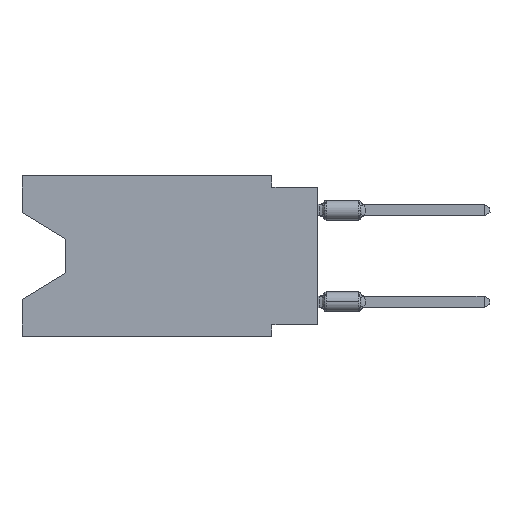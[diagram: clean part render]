
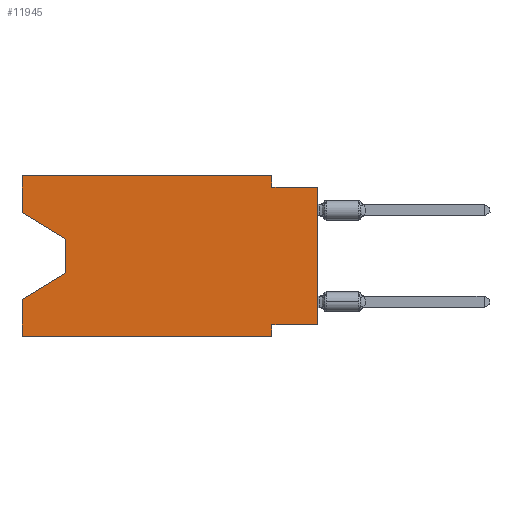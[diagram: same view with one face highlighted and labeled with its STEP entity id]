
A CAD part, left-side view. The second image highlights one B-rep face of the part: STEP entity #11945.
In plain terms, the highlighted planar face has unit normal (-1, 0, 0).
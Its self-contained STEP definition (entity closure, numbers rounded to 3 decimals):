
#227 = VERTEX_POINT ( 'NONE', #22464 ) ;
#343 = VECTOR ( 'NONE', #11981, 1000. ) ;
#1272 = LINE ( 'NONE', #13724, #18395 ) ;
#1464 = CARTESIAN_POINT ( 'NONE',  ( 0., 2.54, -8.255 ) ) ;
#1470 = DIRECTION ( 'NONE',  ( 0., -1., 0. ) ) ;
#1508 = VECTOR ( 'NONE', #5732, 1000. ) ;
#1556 = ORIENTED_EDGE ( 'NONE', *, *, #2219, .F. ) ;
#1916 = EDGE_CURVE ( 'NONE', #15189, #8609, #19212, .T. ) ;
#2058 = LINE ( 'NONE', #9083, #20916 ) ;
#2219 = EDGE_CURVE ( 'NONE', #227, #12542, #18964, .T. ) ;
#2489 = CARTESIAN_POINT ( 'NONE',  ( 0., 2.54, -0.635 ) ) ;
#2504 = LINE ( 'NONE', #8159, #2540 ) ;
#2540 = VECTOR ( 'NONE', #15192, 1000. ) ;
#2694 = VECTOR ( 'NONE', #19600, 1000. ) ;
#3168 = CARTESIAN_POINT ( 'NONE',  ( 0., 16.383, 0. ) ) ;
#3346 = DIRECTION ( 'NONE',  ( 0., 1., 0. ) ) ;
#3397 = DIRECTION ( 'NONE',  ( 0., 0.855, -0.519 ) ) ;
#3561 = CARTESIAN_POINT ( 'NONE',  ( 0., 0., -0.635 ) ) ;
#3777 = CARTESIAN_POINT ( 'NONE',  ( 0., 16.383, -8.89 ) ) ;
#4109 = CARTESIAN_POINT ( 'NONE',  ( 0., 2.54, -8.89 ) ) ;
#4114 = CARTESIAN_POINT ( 'NONE',  ( 0., 16.383, -2.038 ) ) ;
#4242 = CARTESIAN_POINT ( 'NONE',  ( 0., 0., -8.255 ) ) ;
#4996 = VERTEX_POINT ( 'NONE', #4109 ) ;
#5250 = ORIENTED_EDGE ( 'NONE', *, *, #13759, .F. ) ;
#5732 = DIRECTION ( 'NONE',  ( 0., -1., 0. ) ) ;
#5753 = CARTESIAN_POINT ( 'NONE',  ( 0., 16.383, -6.852 ) ) ;
#6162 = CARTESIAN_POINT ( 'NONE',  ( 0., 13.97, -5.385 ) ) ;
#6175 = PLANE ( 'NONE',  #8049 ) ;
#6365 = VERTEX_POINT ( 'NONE', #2489 ) ;
#6407 = DIRECTION ( 'NONE',  ( 0., 0., 1. ) ) ;
#6963 = VECTOR ( 'NONE', #1470, 1000. ) ;
#7028 = LINE ( 'NONE', #21099, #15801 ) ;
#7045 = EDGE_CURVE ( 'NONE', #15189, #11457, #2058, .T. ) ;
#7484 = DIRECTION ( 'NONE',  ( 0., 0., 1. ) ) ;
#7676 = DIRECTION ( 'NONE',  ( 1., 0., 0. ) ) ;
#8006 = CARTESIAN_POINT ( 'NONE',  ( 0., 0., -0.635 ) ) ;
#8049 = AXIS2_PLACEMENT_3D ( 'NONE', #14593, #7676, #16686 ) ;
#8159 = CARTESIAN_POINT ( 'NONE',  ( 0., 2.54, -8.89 ) ) ;
#8609 = VERTEX_POINT ( 'NONE', #9090 ) ;
#9083 = CARTESIAN_POINT ( 'NONE',  ( 0., 16.383, 0. ) ) ;
#9090 = CARTESIAN_POINT ( 'NONE',  ( 0., 13.97, -3.505 ) ) ;
#9149 = CARTESIAN_POINT ( 'NONE',  ( 0., 13.97, -3.505 ) ) ;
#9160 = ORIENTED_EDGE ( 'NONE', *, *, #18349, .T. ) ;
#9406 = LINE ( 'NONE', #3777, #1508 ) ;
#10370 = LINE ( 'NONE', #3561, #343 ) ;
#10727 = LINE ( 'NONE', #21787, #2694 ) ;
#10815 = ORIENTED_EDGE ( 'NONE', *, *, #7045, .F. ) ;
#11188 = EDGE_CURVE ( 'NONE', #11465, #11689, #1272, .T. ) ;
#11203 = EDGE_CURVE ( 'NONE', #6365, #21708, #10370, .T. ) ;
#11457 = VERTEX_POINT ( 'NONE', #20043 ) ;
#11465 = VERTEX_POINT ( 'NONE', #4242 ) ;
#11689 = VERTEX_POINT ( 'NONE', #1464 ) ;
#11945 = ADVANCED_FACE ( 'NONE', ( #13098 ), #6175, .F. ) ;
#11981 = DIRECTION ( 'NONE',  ( 0., -1., 0. ) ) ;
#12382 = EDGE_CURVE ( 'NONE', #17687, #6365, #7028, .T. ) ;
#12542 = VERTEX_POINT ( 'NONE', #5753 ) ;
#12720 = ORIENTED_EDGE ( 'NONE', *, *, #11203, .F. ) ;
#13098 = FACE_OUTER_BOUND ( 'NONE', #14072, .T. ) ;
#13263 = VECTOR ( 'NONE', #3397, 1000. ) ;
#13280 = ORIENTED_EDGE ( 'NONE', *, *, #11188, .F. ) ;
#13308 = VECTOR ( 'NONE', #13913, 1000. ) ;
#13724 = CARTESIAN_POINT ( 'NONE',  ( 0., 0., -8.255 ) ) ;
#13759 = EDGE_CURVE ( 'NONE', #11457, #17687, #15653, .T. ) ;
#13913 = DIRECTION ( 'NONE',  ( 0., -0.855, -0.519 ) ) ;
#14072 = EDGE_LOOP ( 'NONE', ( #15788, #9160, #15141, #1556, #22695, #16688, #13280, #14686, #12720, #17337, #5250, #10815 ) ) ;
#14593 = CARTESIAN_POINT ( 'NONE',  ( 0., 16.383, 0. ) ) ;
#14686 = ORIENTED_EDGE ( 'NONE', *, *, #19198, .T. ) ;
#14922 = DIRECTION ( 'NONE',  ( 0., 0., -1. ) ) ;
#15141 = ORIENTED_EDGE ( 'NONE', *, *, #21899, .T. ) ;
#15189 = VERTEX_POINT ( 'NONE', #4114 ) ;
#15192 = DIRECTION ( 'NONE',  ( 0., 0., -1. ) ) ;
#15242 = EDGE_CURVE ( 'NONE', #227, #4996, #9406, .T. ) ;
#15545 = VECTOR ( 'NONE', #14922, 1000. ) ;
#15653 = LINE ( 'NONE', #20620, #6963 ) ;
#15788 = ORIENTED_EDGE ( 'NONE', *, *, #1916, .T. ) ;
#15801 = VECTOR ( 'NONE', #19021, 1000. ) ;
#15867 = CARTESIAN_POINT ( 'NONE',  ( 0., 16.383, -2.038 ) ) ;
#16327 = LINE ( 'NONE', #9149, #15545 ) ;
#16686 = DIRECTION ( 'NONE',  ( 0., 0., -1. ) ) ;
#16688 = ORIENTED_EDGE ( 'NONE', *, *, #20996, .F. ) ;
#17128 = VERTEX_POINT ( 'NONE', #6162 ) ;
#17282 = CARTESIAN_POINT ( 'NONE',  ( 0., 2.54, 0. ) ) ;
#17337 = ORIENTED_EDGE ( 'NONE', *, *, #12382, .F. ) ;
#17687 = VERTEX_POINT ( 'NONE', #17282 ) ;
#18349 = EDGE_CURVE ( 'NONE', #8609, #17128, #16327, .T. ) ;
#18395 = VECTOR ( 'NONE', #3346, 1000. ) ;
#18520 = VECTOR ( 'NONE', #6407, 1000. ) ;
#18964 = LINE ( 'NONE', #3168, #18520 ) ;
#19021 = DIRECTION ( 'NONE',  ( 0., 0., -1. ) ) ;
#19198 = EDGE_CURVE ( 'NONE', #11465, #21708, #10727, .T. ) ;
#19212 = LINE ( 'NONE', #15867, #13308 ) ;
#19600 = DIRECTION ( 'NONE',  ( 0., 0., 1. ) ) ;
#20043 = CARTESIAN_POINT ( 'NONE',  ( 0., 16.383, 0. ) ) ;
#20579 = CARTESIAN_POINT ( 'NONE',  ( 0., 13.97, -5.385 ) ) ;
#20620 = CARTESIAN_POINT ( 'NONE',  ( 0., 16.383, 0. ) ) ;
#20802 = LINE ( 'NONE', #20579, #13263 ) ;
#20916 = VECTOR ( 'NONE', #7484, 1000. ) ;
#20996 = EDGE_CURVE ( 'NONE', #11689, #4996, #2504, .T. ) ;
#21099 = CARTESIAN_POINT ( 'NONE',  ( 0., 2.54, 0. ) ) ;
#21708 = VERTEX_POINT ( 'NONE', #8006 ) ;
#21787 = CARTESIAN_POINT ( 'NONE',  ( 0., 0., 0. ) ) ;
#21899 = EDGE_CURVE ( 'NONE', #17128, #12542, #20802, .T. ) ;
#22464 = CARTESIAN_POINT ( 'NONE',  ( 0., 16.383, -8.89 ) ) ;
#22695 = ORIENTED_EDGE ( 'NONE', *, *, #15242, .T. ) ;
